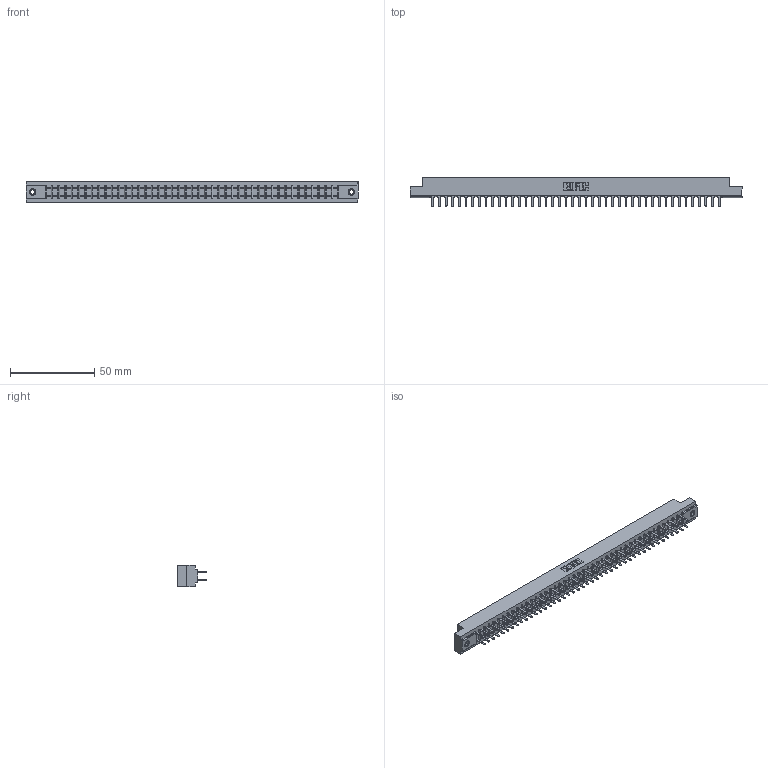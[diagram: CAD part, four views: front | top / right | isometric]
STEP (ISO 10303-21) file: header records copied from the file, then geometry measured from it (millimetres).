
FILE_DESCRIPTION (( 'STEP AP203' ), '1' );
FILE_NAME ('807-088-520-207.STEP', '2021-07-20T20:41:22', ( '' ), ( '' ), 'SwSTEP 2.0', 'SolidWorks 2020', '' );
FILE_SCHEMA (( 'CONFIG_CONTROL_DESIGN' ));
Length unit declared in the file: inch
Products named in the file (4): 307-290-001_520; 345-250-001_345-250-005-103; 807-088-520-207; 807 Part_.156 Dia Mounting Holes
Assembly tree (91 placements, depth 2):
  807-088-520-207
    807 Part_.156 Dia Mounting Holes
    307-290-001_520  x88
    345-250-001_345-250-005-103  x2
Bounding box: 197.36 x 17.42 x 12.7 mm (x, y, z)
Volume: 21051.9 mm3; surface area: 25973.2 mm2
Topology: 91 solids, 91 shells, 4271 faces, 11899 edges, 7686 vertices
Faces by surface type: plane 2830, cylinder 1335, sphere 90, cone 12, torus 4
Entity records: 40035 total; most frequent: CARTESIAN_POINT 6531, ORIENTED_EDGE 6466, DIRECTION 6405, EDGE_CURVE 3233, VECTOR 2481, LINE 2481, VERTEX_POINT 2088, AXIS2_PLACEMENT_3D 1962
